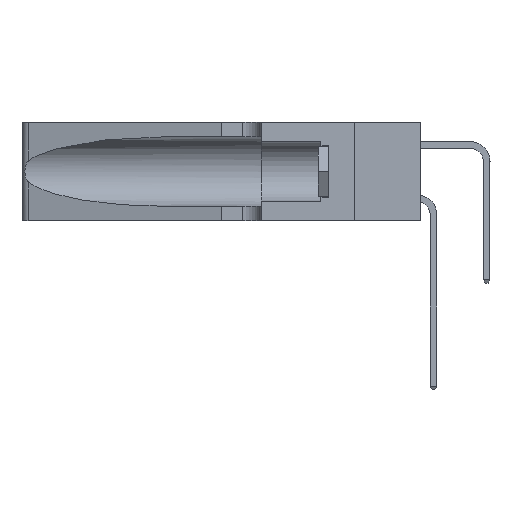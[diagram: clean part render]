
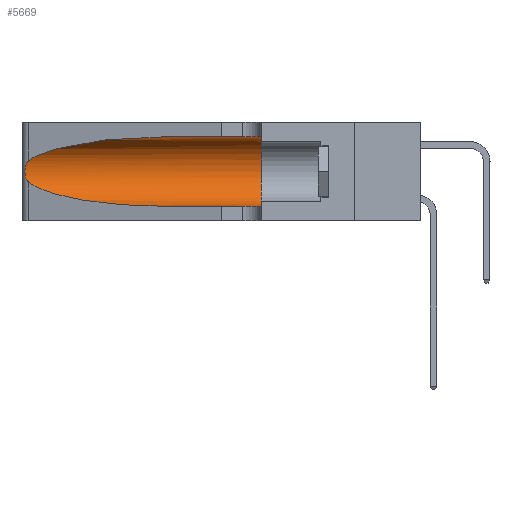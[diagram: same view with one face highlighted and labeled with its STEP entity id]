
A CAD part, left-side view. The second image highlights one B-rep face of the part: STEP entity #5669.
In plain terms, the highlighted cylindrical face has radius 3.308 mm (diameter 6.617 mm), a partial arc.
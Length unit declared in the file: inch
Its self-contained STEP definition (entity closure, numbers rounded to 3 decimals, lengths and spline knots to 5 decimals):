
#1154 = CARTESIAN_POINT ( 'NONE',  ( 0.2373, 1.15595, 0.28018 ) ) ;
#1322 = VERTEX_POINT ( 'NONE', #15921 ) ;
#1546 = EDGE_LOOP ( 'NONE', ( #2228, #20033, #20721, #28672, #7463, #10519 ) ) ;
#1672 = CARTESIAN_POINT ( 'NONE',  ( 0.25787, 1.23484, 0.2124 ) ) ;
#2228 = ORIENTED_EDGE ( 'NONE', *, *, #21666, .T. ) ;
#3957 = CARTESIAN_POINT ( 'NONE',  ( 0.1305, 0.72297, 0.31525 ) ) ;
#4018 = CARTESIAN_POINT ( 'NONE',  ( 0.2373, 1.15595, 0.08982 ) ) ;
#4251 = LINE ( 'NONE', #15256, #19410 ) ;
#4857 = CARTESIAN_POINT ( 'NONE',  ( 0.1305, 0.72297, 0.31525 ) ) ;
#5669 = ADVANCED_FACE ( 'NONE', ( #6981 ), #20451, .F. ) ;
#6303 = AXIS2_PLACEMENT_3D ( 'NONE', #12230, #33828, #7180 ) ;
#6444 =( BOUNDED_CURVE ( )  B_SPLINE_CURVE ( 3, ( #30687, #4018, #25419, #6486 ),
 .UNSPECIFIED., .F., .F. ) 
 B_SPLINE_CURVE_WITH_KNOTS ( ( 4, 4 ),
 ( 3.44316, 4.71239 ),
 .UNSPECIFIED. ) 
 CURVE ( )  GEOMETRIC_REPRESENTATION_ITEM ( )  RATIONAL_B_SPLINE_CURVE ( ( 1., 0.87, 0.87, 1. ) ) 
 REPRESENTATION_ITEM ( '' )  );
#6486 = CARTESIAN_POINT ( 'NONE',  ( 0.1305, 0.72297, 0.05475 ) ) ;
#6864 = AXIS2_PLACEMENT_3D ( 'NONE', #27952, #9319, #14598 ) ;
#6981 = FACE_OUTER_BOUND ( 'NONE', #1546, .T. ) ;
#7138 = CARTESIAN_POINT ( 'NONE',  ( 0.26017, 1.23833, 0.17102 ) ) ;
#7180 = DIRECTION ( 'NONE',  ( 0., 0., -1. ) ) ;
#7258 = CARTESIAN_POINT ( 'NONE',  ( 0.25639, 1.23184, 0.21858 ) ) ;
#7463 = ORIENTED_EDGE ( 'NONE', *, *, #32585, .F. ) ;
#7512 = CARTESIAN_POINT ( 'NONE',  ( 0.25555, 1.22993, 0.14849 ) ) ;
#8817 = CARTESIAN_POINT ( 'NONE',  ( 0.1305, 0.35, 0.31525 ) ) ;
#9319 = DIRECTION ( 'NONE',  ( 0., 1., 0. ) ) ;
#9338 = CARTESIAN_POINT ( 'NONE',  ( 0.1305, 0.35, 0.05475 ) ) ;
#10519 = ORIENTED_EDGE ( 'NONE', *, *, #16270, .F. ) ;
#10686 = LINE ( 'NONE', #30657, #11859 ) ;
#11859 = VECTOR ( 'NONE', #17060, 39.37008 ) ;
#12087 = VERTEX_POINT ( 'NONE', #4857 ) ;
#12230 = CARTESIAN_POINT ( 'NONE',  ( 0.1305, 1.61858, 0.185 ) ) ;
#14032 = VERTEX_POINT ( 'NONE', #8817 ) ;
#14429 = CARTESIAN_POINT ( 'NONE',  ( 0.18966, 0.96281, 0.31525 ) ) ;
#14598 = DIRECTION ( 'NONE',  ( 0., 0., 1. ) ) ;
#14744 = VERTEX_POINT ( 'NONE', #9338 ) ;
#15117 = CARTESIAN_POINT ( 'NONE',  ( 0.25487, 1.22718, 0.22369 ) ) ;
#15256 = CARTESIAN_POINT ( 'NONE',  ( 0.1305, 1.61858, 0.31525 ) ) ;
#15921 = CARTESIAN_POINT ( 'NONE',  ( 0.1305, 0.72297, 0.05475 ) ) ;
#16270 = EDGE_CURVE ( 'NONE', #12087, #14032, #4251, .T. ) ;
#17060 = DIRECTION ( 'NONE',  ( 0., -1., 0. ) ) ;
#17467 = CARTESIAN_POINT ( 'NONE',  ( 0.25639, 1.23186, 0.15144 ) ) ;
#17964 = CARTESIAN_POINT ( 'NONE',  ( 0.25856, 1.23593, 0.16098 ) ) ;
#18467 = EDGE_CURVE ( 'NONE', #28511, #1322, #6444, .T. ) ;
#19407 = B_SPLINE_CURVE_WITH_KNOTS ( 'NONE', 3,
 ( #15117, #33902, #7258, #1672, #31313, #34024, #23237, #33532, #7138, #17964, #30835, #17467, #7512, #21018 ),
 .UNSPECIFIED., .F., .F.,
 ( 4, 2, 2, 2, 2, 2, 4 ),
 ( 0., 0.00027, 0.00053, 0.00107, 0.0016, 0.00187, 0.00214 ),
 .UNSPECIFIED. ) ;
#19410 = VECTOR ( 'NONE', #29106, 39.37008 ) ;
#20033 = ORIENTED_EDGE ( 'NONE', *, *, #30468, .T. ) ;
#20451 = CYLINDRICAL_SURFACE ( 'NONE', #6303, 0.13025 ) ;
#20721 = ORIENTED_EDGE ( 'NONE', *, *, #18467, .T. ) ;
#21018 = CARTESIAN_POINT ( 'NONE',  ( 0.25487, 1.22718, 0.14631 ) ) ;
#21666 = EDGE_CURVE ( 'NONE', #12087, #28644, #27751, .T. ) ;
#23237 = CARTESIAN_POINT ( 'NONE',  ( 0.26075, 1.23896, 0.19203 ) ) ;
#24302 = EDGE_CURVE ( 'NONE', #1322, #14744, #10686, .T. ) ;
#25419 = CARTESIAN_POINT ( 'NONE',  ( 0.18966, 0.96281, 0.05475 ) ) ;
#27751 =( BOUNDED_CURVE ( )  B_SPLINE_CURVE ( 3, ( #3957, #14429, #1154, #34391 ),
 .UNSPECIFIED., .F., .F. ) 
 B_SPLINE_CURVE_WITH_KNOTS ( ( 4, 4 ),
 ( 1.5708, 2.84003 ),
 .UNSPECIFIED. ) 
 CURVE ( )  GEOMETRIC_REPRESENTATION_ITEM ( )  RATIONAL_B_SPLINE_CURVE ( ( 1., 0.87, 0.87, 1. ) ) 
 REPRESENTATION_ITEM ( '' )  );
#27952 = CARTESIAN_POINT ( 'NONE',  ( 0.1305, 0.35, 0.185 ) ) ;
#28511 = VERTEX_POINT ( 'NONE', #29353 ) ;
#28644 = VERTEX_POINT ( 'NONE', #28796 ) ;
#28672 = ORIENTED_EDGE ( 'NONE', *, *, #24302, .T. ) ;
#28796 = CARTESIAN_POINT ( 'NONE',  ( 0.25487, 1.22718, 0.22369 ) ) ;
#29106 = DIRECTION ( 'NONE',  ( 0., -1., 0. ) ) ;
#29353 = CARTESIAN_POINT ( 'NONE',  ( 0.25487, 1.22718, 0.14631 ) ) ;
#29720 = CIRCLE ( 'NONE', #6864, 0.13025 ) ;
#30468 = EDGE_CURVE ( 'NONE', #28644, #28511, #19407, .T. ) ;
#30657 = CARTESIAN_POINT ( 'NONE',  ( 0.1305, 1.61858, 0.05475 ) ) ;
#30687 = CARTESIAN_POINT ( 'NONE',  ( 0.25487, 1.22718, 0.14631 ) ) ;
#30835 = CARTESIAN_POINT ( 'NONE',  ( 0.25789, 1.23486, 0.15765 ) ) ;
#31313 = CARTESIAN_POINT ( 'NONE',  ( 0.25854, 1.2359, 0.20912 ) ) ;
#32585 = EDGE_CURVE ( 'NONE', #14032, #14744, #29720, .T. ) ;
#33532 = CARTESIAN_POINT ( 'NONE',  ( 0.26075, 1.23896, 0.178 ) ) ;
#33828 = DIRECTION ( 'NONE',  ( 0., -1., 0. ) ) ;
#33902 = CARTESIAN_POINT ( 'NONE',  ( 0.25555, 1.22994, 0.2215 ) ) ;
#34024 = CARTESIAN_POINT ( 'NONE',  ( 0.26018, 1.23835, 0.19895 ) ) ;
#34391 = CARTESIAN_POINT ( 'NONE',  ( 0.25487, 1.22718, 0.22369 ) ) ;
